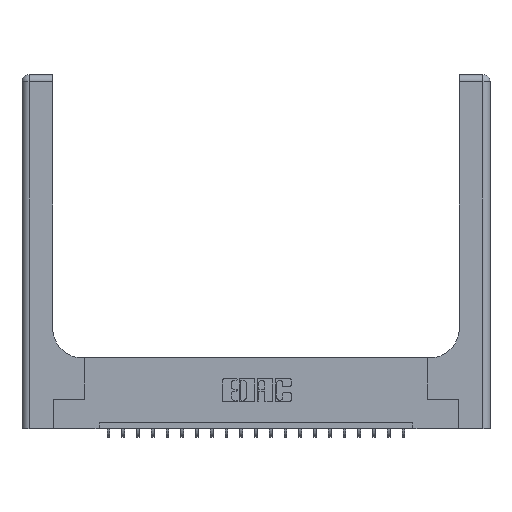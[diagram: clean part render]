
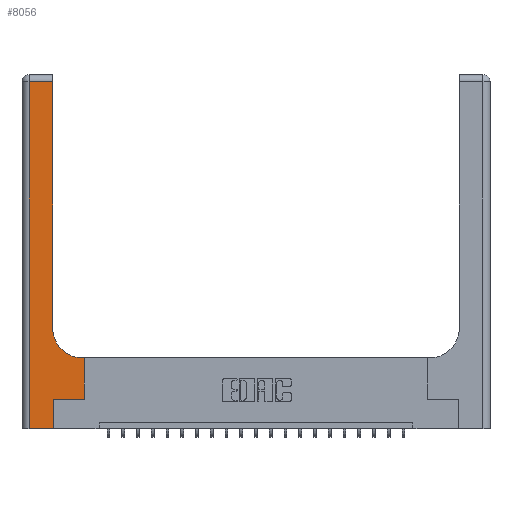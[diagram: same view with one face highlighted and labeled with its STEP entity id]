
A CAD part, top view. The second image highlights one B-rep face of the part: STEP entity #8056.
In plain terms, the highlighted planar face has unit normal (0, 0, 1).
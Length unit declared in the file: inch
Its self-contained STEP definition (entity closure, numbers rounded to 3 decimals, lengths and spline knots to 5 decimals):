
#133 = DIRECTION ( 'NONE',  ( 0., 1., 0. ) ) ;
#176 = CARTESIAN_POINT ( 'NONE',  ( 0.06, 3., 0.37 ) ) ;
#270 = VERTEX_POINT ( 'NONE', #2310 ) ;
#440 = ORIENTED_EDGE ( 'NONE', *, *, #2846, .T. ) ;
#556 = AXIS2_PLACEMENT_3D ( 'NONE', #18348, #8603, #19955 ) ;
#983 = ORIENTED_EDGE ( 'NONE', *, *, #10782, .T. ) ;
#1107 = ORIENTED_EDGE ( 'NONE', *, *, #20816, .T. ) ;
#2310 = CARTESIAN_POINT ( 'NONE',  ( 0.265, 0.25, 0.37 ) ) ;
#2679 = DIRECTION ( 'NONE',  ( 0., 1., 0. ) ) ;
#2720 = VERTEX_POINT ( 'NONE', #3533 ) ;
#2846 = EDGE_CURVE ( 'NONE', #2720, #14809, #11517, .T. ) ;
#3015 = LINE ( 'NONE', #19422, #7887 ) ;
#3231 = VERTEX_POINT ( 'NONE', #11320 ) ;
#3397 = EDGE_CURVE ( 'NONE', #14809, #5674, #10481, .T. ) ;
#3533 = CARTESIAN_POINT ( 'NONE',  ( 0.528, 0.6, 0.37 ) ) ;
#3614 = VECTOR ( 'NONE', #11669, 39.37008 ) ;
#3810 = DIRECTION ( 'NONE',  ( -1., 0., 0. ) ) ;
#4413 = DIRECTION ( 'NONE',  ( -1., 0., 0. ) ) ;
#4437 = VECTOR ( 'NONE', #133, 39.37008 ) ;
#4593 = DIRECTION ( 'NONE',  ( 0., 1., 0. ) ) ;
#4718 = CARTESIAN_POINT ( 'NONE',  ( 0.265, 0.25, 0.37 ) ) ;
#5398 = LINE ( 'NONE', #15824, #10263 ) ;
#5404 = CARTESIAN_POINT ( 'NONE',  ( 0.26, 0.6, 0.37 ) ) ;
#5674 = VERTEX_POINT ( 'NONE', #6702 ) ;
#6015 = VERTEX_POINT ( 'NONE', #15817 ) ;
#6614 = VERTEX_POINT ( 'NONE', #9599 ) ;
#6702 = CARTESIAN_POINT ( 'NONE',  ( 0.26, 0.85, 0.37 ) ) ;
#7167 = VECTOR ( 'NONE', #3810, 39.37008 ) ;
#7352 = CARTESIAN_POINT ( 'NONE',  ( 0.06, 0., 0.37 ) ) ;
#7443 = VECTOR ( 'NONE', #14485, 39.37008 ) ;
#7886 = ORIENTED_EDGE ( 'NONE', *, *, #17243, .T. ) ;
#7887 = VECTOR ( 'NONE', #8047, 39.37008 ) ;
#8047 = DIRECTION ( 'NONE',  ( 1., 0., 0. ) ) ;
#8056 = ADVANCED_FACE ( 'NONE', ( #16669 ), #11196, .F. ) ;
#8603 = DIRECTION ( 'NONE',  ( 0., 0., -1. ) ) ;
#8760 = VERTEX_POINT ( 'NONE', #7352 ) ;
#9599 = CARTESIAN_POINT ( 'NONE',  ( 0.528, 0.25, 0.37 ) ) ;
#9611 = DIRECTION ( 'NONE',  ( 0., 0., -1. ) ) ;
#10073 = ORIENTED_EDGE ( 'NONE', *, *, #11450, .T. ) ;
#10263 = VECTOR ( 'NONE', #4413, 39.37008 ) ;
#10481 = CIRCLE ( 'NONE', #556, 0.25 ) ;
#10782 = EDGE_CURVE ( 'NONE', #8760, #13276, #3015, .T. ) ;
#10850 = CARTESIAN_POINT ( 'NONE',  ( 0.26, 3., 0.37 ) ) ;
#10865 = CARTESIAN_POINT ( 'NONE',  ( 0.51, 0.6, 0.37 ) ) ;
#11196 = PLANE ( 'NONE',  #16392 ) ;
#11320 = CARTESIAN_POINT ( 'NONE',  ( 0.06, 2.94, 0.37 ) ) ;
#11450 = EDGE_CURVE ( 'NONE', #6614, #2720, #21040, .T. ) ;
#11517 = LINE ( 'NONE', #5404, #7167 ) ;
#11624 = CARTESIAN_POINT ( 'NONE',  ( 0.265, 0., 0.37 ) ) ;
#11669 = DIRECTION ( 'NONE',  ( 0., -1., 0. ) ) ;
#11777 = LINE ( 'NONE', #4718, #7443 ) ;
#12307 = LINE ( 'NONE', #176, #3614 ) ;
#12434 = VECTOR ( 'NONE', #4593, 39.37008 ) ;
#13136 = EDGE_LOOP ( 'NONE', ( #1107, #20660, #19989, #983, #14665, #7886, #10073, #440, #13446 ) ) ;
#13276 = VERTEX_POINT ( 'NONE', #18165 ) ;
#13446 = ORIENTED_EDGE ( 'NONE', *, *, #3397, .T. ) ;
#14441 = CARTESIAN_POINT ( 'NONE',  ( 0., 3., 0.37 ) ) ;
#14485 = DIRECTION ( 'NONE',  ( 1., 0., 0. ) ) ;
#14665 = ORIENTED_EDGE ( 'NONE', *, *, #16083, .T. ) ;
#14809 = VERTEX_POINT ( 'NONE', #10865 ) ;
#15817 = CARTESIAN_POINT ( 'NONE',  ( 0.26, 2.94, 0.37 ) ) ;
#15824 = CARTESIAN_POINT ( 'NONE',  ( 0., 2.94, 0.37 ) ) ;
#16008 = CARTESIAN_POINT ( 'NONE',  ( 0.528, 0.25, 0.37 ) ) ;
#16083 = EDGE_CURVE ( 'NONE', #13276, #270, #16418, .T. ) ;
#16122 = VECTOR ( 'NONE', #2679, 39.37008 ) ;
#16392 = AXIS2_PLACEMENT_3D ( 'NONE', #14441, #9611, #20940 ) ;
#16418 = LINE ( 'NONE', #11624, #4437 ) ;
#16669 = FACE_OUTER_BOUND ( 'NONE', #13136, .T. ) ;
#16783 = EDGE_CURVE ( 'NONE', #3231, #8760, #12307, .T. ) ;
#17243 = EDGE_CURVE ( 'NONE', #270, #6614, #11777, .T. ) ;
#18165 = CARTESIAN_POINT ( 'NONE',  ( 0.265, 0., 0.37 ) ) ;
#18348 = CARTESIAN_POINT ( 'NONE',  ( 0.51, 0.85, 0.37 ) ) ;
#19422 = CARTESIAN_POINT ( 'NONE',  ( 0., 0., 0.37 ) ) ;
#19902 = LINE ( 'NONE', #10850, #16122 ) ;
#19955 = DIRECTION ( 'NONE',  ( 1., 0., 0. ) ) ;
#19989 = ORIENTED_EDGE ( 'NONE', *, *, #16783, .T. ) ;
#20660 = ORIENTED_EDGE ( 'NONE', *, *, #20856, .T. ) ;
#20816 = EDGE_CURVE ( 'NONE', #5674, #6015, #19902, .T. ) ;
#20856 = EDGE_CURVE ( 'NONE', #6015, #3231, #5398, .T. ) ;
#20940 = DIRECTION ( 'NONE',  ( -1., 0., 0. ) ) ;
#21040 = LINE ( 'NONE', #16008, #12434 ) ;
